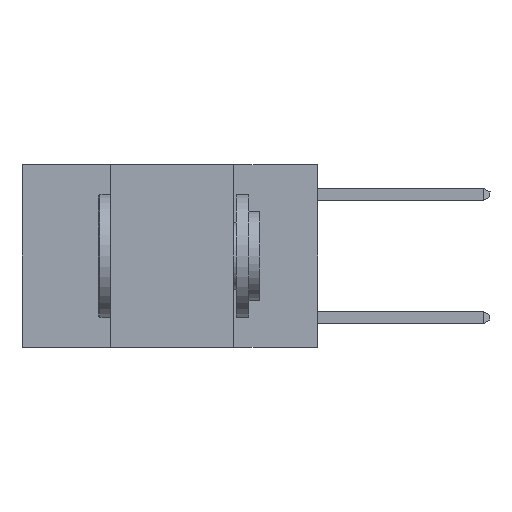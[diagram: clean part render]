
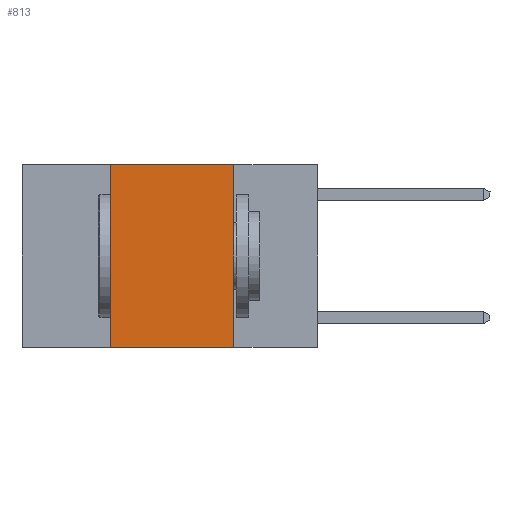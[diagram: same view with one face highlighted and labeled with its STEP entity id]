
A CAD part, left-side view. The second image highlights one B-rep face of the part: STEP entity #813.
In plain terms, the highlighted planar face has unit normal (-1, 0, 0).
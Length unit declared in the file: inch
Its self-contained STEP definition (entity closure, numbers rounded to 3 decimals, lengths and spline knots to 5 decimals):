
#87 = VERTEX_POINT ( 'NONE', #10485 ) ;
#250 = CARTESIAN_POINT ( 'NONE',  ( 0., 0.42, 0. ) ) ;
#439 = CARTESIAN_POINT ( 'NONE',  ( 0., 0.17, 0. ) ) ;
#677 = CARTESIAN_POINT ( 'NONE',  ( 0., 0.6, 0. ) ) ;
#813 = ADVANCED_FACE ( 'NONE', ( #9272 ), #10451, .F. ) ;
#892 = CARTESIAN_POINT ( 'NONE',  ( 0., 0.17, 0. ) ) ;
#1147 = VECTOR ( 'NONE', #8659, 39.37008 ) ;
#1272 = VERTEX_POINT ( 'NONE', #250 ) ;
#1425 = LINE ( 'NONE', #677, #1147 ) ;
#1480 = CARTESIAN_POINT ( 'NONE',  ( 0., 0.6, 0. ) ) ;
#2384 = CARTESIAN_POINT ( 'NONE',  ( 0., 0.42, 0. ) ) ;
#2580 = DIRECTION ( 'NONE',  ( 0., -1., 0. ) ) ;
#3182 = DIRECTION ( 'NONE',  ( 0., 0., 1. ) ) ;
#3473 = LINE ( 'NONE', #2384, #9553 ) ;
#3663 = ORIENTED_EDGE ( 'NONE', *, *, #5319, .T. ) ;
#3835 = CARTESIAN_POINT ( 'NONE',  ( 0., 0.42, -0.37 ) ) ;
#4103 = VECTOR ( 'NONE', #2580, 39.37008 ) ;
#4288 = LINE ( 'NONE', #439, #10612 ) ;
#4430 = EDGE_CURVE ( 'NONE', #1272, #6380, #1425, .T. ) ;
#4837 = ORIENTED_EDGE ( 'NONE', *, *, #8841, .F. ) ;
#4967 = AXIS2_PLACEMENT_3D ( 'NONE', #1480, #10319, #10316 ) ;
#5110 = EDGE_CURVE ( 'NONE', #6810, #1272, #3473, .T. ) ;
#5319 = EDGE_CURVE ( 'NONE', #6810, #87, #10170, .T. ) ;
#6244 = DIRECTION ( 'NONE',  ( 0., 0., -1. ) ) ;
#6380 = VERTEX_POINT ( 'NONE', #892 ) ;
#6810 = VERTEX_POINT ( 'NONE', #3835 ) ;
#8156 = CARTESIAN_POINT ( 'NONE',  ( 0., 0.6, -0.37 ) ) ;
#8187 = ORIENTED_EDGE ( 'NONE', *, *, #4430, .F. ) ;
#8659 = DIRECTION ( 'NONE',  ( 0., -1., 0. ) ) ;
#8841 = EDGE_CURVE ( 'NONE', #6380, #87, #4288, .T. ) ;
#9106 = ORIENTED_EDGE ( 'NONE', *, *, #5110, .F. ) ;
#9272 = FACE_OUTER_BOUND ( 'NONE', #9691, .T. ) ;
#9553 = VECTOR ( 'NONE', #3182, 39.37008 ) ;
#9691 = EDGE_LOOP ( 'NONE', ( #4837, #8187, #9106, #3663 ) ) ;
#10170 = LINE ( 'NONE', #8156, #4103 ) ;
#10316 = DIRECTION ( 'NONE',  ( 0., 0., -1. ) ) ;
#10319 = DIRECTION ( 'NONE',  ( 1., 0., 0. ) ) ;
#10451 = PLANE ( 'NONE',  #4967 ) ;
#10485 = CARTESIAN_POINT ( 'NONE',  ( 0., 0.17, -0.37 ) ) ;
#10612 = VECTOR ( 'NONE', #6244, 39.37008 ) ;
